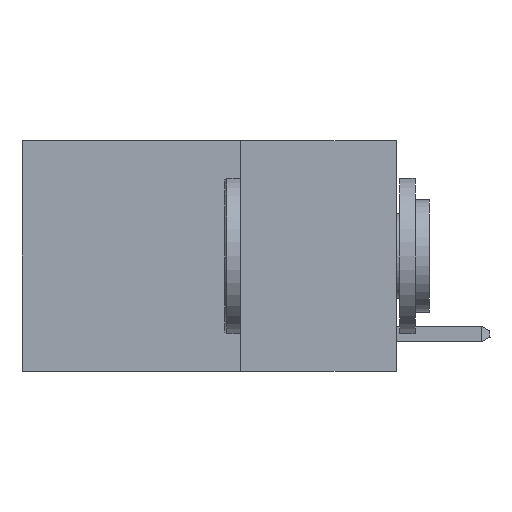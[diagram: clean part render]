
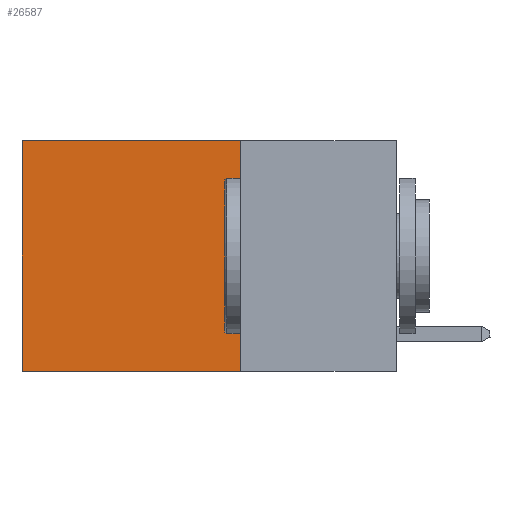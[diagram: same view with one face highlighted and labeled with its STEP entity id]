
A CAD part, left-side view. The second image highlights one B-rep face of the part: STEP entity #26587.
In plain terms, the highlighted planar face has unit normal (-1, 0, 0).
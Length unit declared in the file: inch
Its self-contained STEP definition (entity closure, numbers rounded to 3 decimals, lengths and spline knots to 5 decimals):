
#540 = VERTEX_POINT ( 'NONE', #3942 ) ;
#833 = EDGE_CURVE ( 'NONE', #18436, #19555, #4717, .T. ) ;
#1367 = DIRECTION ( 'NONE',  ( 1., 0., 0. ) ) ;
#1503 = DIRECTION ( 'NONE',  ( 0., 0., -1. ) ) ;
#2138 = ORIENTED_EDGE ( 'NONE', *, *, #26562, .T. ) ;
#2438 = EDGE_CURVE ( 'NONE', #540, #27247, #3573, .T. ) ;
#3573 = LINE ( 'NONE', #11887, #20135 ) ;
#3867 = CARTESIAN_POINT ( 'NONE',  ( 0.2625, 0.25, 0. ) ) ;
#3942 = CARTESIAN_POINT ( 'NONE',  ( 0.2625, 0.6, 0. ) ) ;
#4717 = LINE ( 'NONE', #23959, #27924 ) ;
#5576 = VECTOR ( 'NONE', #28305, 39.37008 ) ;
#10264 = CARTESIAN_POINT ( 'NONE',  ( 0.2625, 0.25, 0. ) ) ;
#11587 = LINE ( 'NONE', #26082, #5576 ) ;
#11887 = CARTESIAN_POINT ( 'NONE',  ( 0.2625, 0.6, 0. ) ) ;
#11985 = ORIENTED_EDGE ( 'NONE', *, *, #833, .F. ) ;
#12508 = DIRECTION ( 'NONE',  ( 0., 1., 0. ) ) ;
#12689 = AXIS2_PLACEMENT_3D ( 'NONE', #28200, #1367, #17113 ) ;
#13604 = CARTESIAN_POINT ( 'NONE',  ( 0.2625, 0.25, -0.37 ) ) ;
#14862 = PLANE ( 'NONE',  #12689 ) ;
#15787 = FACE_OUTER_BOUND ( 'NONE', #16813, .T. ) ;
#16481 = VECTOR ( 'NONE', #12508, 39.37008 ) ;
#16813 = EDGE_LOOP ( 'NONE', ( #17494, #22403, #11985, #2138 ) ) ;
#17113 = DIRECTION ( 'NONE',  ( 0., 0., -1. ) ) ;
#17494 = ORIENTED_EDGE ( 'NONE', *, *, #2438, .T. ) ;
#18436 = VERTEX_POINT ( 'NONE', #3867 ) ;
#19555 = VERTEX_POINT ( 'NONE', #13604 ) ;
#20135 = VECTOR ( 'NONE', #25358, 39.37008 ) ;
#22403 = ORIENTED_EDGE ( 'NONE', *, *, #28515, .F. ) ;
#22487 = LINE ( 'NONE', #10264, #16481 ) ;
#23775 = CARTESIAN_POINT ( 'NONE',  ( 0.2625, 0.6, -0.37 ) ) ;
#23959 = CARTESIAN_POINT ( 'NONE',  ( 0.2625, 0.25, 0. ) ) ;
#25358 = DIRECTION ( 'NONE',  ( 0., 0., -1. ) ) ;
#26082 = CARTESIAN_POINT ( 'NONE',  ( 0.2625, 0.25, -0.37 ) ) ;
#26562 = EDGE_CURVE ( 'NONE', #18436, #540, #22487, .T. ) ;
#26587 = ADVANCED_FACE ( 'NONE', ( #15787 ), #14862, .F. ) ;
#27247 = VERTEX_POINT ( 'NONE', #23775 ) ;
#27924 = VECTOR ( 'NONE', #1503, 39.37008 ) ;
#28200 = CARTESIAN_POINT ( 'NONE',  ( 0.2625, 0.25, 0. ) ) ;
#28305 = DIRECTION ( 'NONE',  ( 0., 1., 0. ) ) ;
#28515 = EDGE_CURVE ( 'NONE', #19555, #27247, #11587, .T. ) ;
